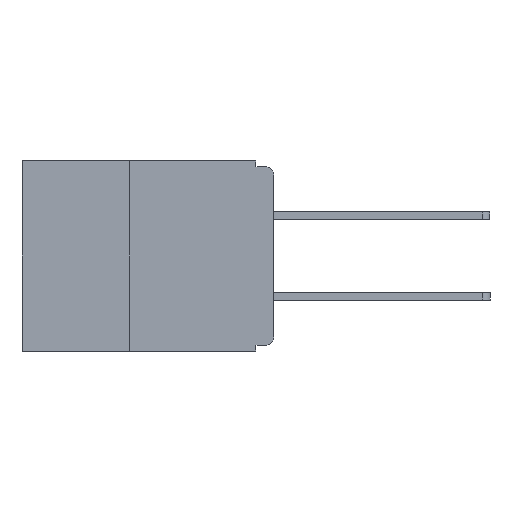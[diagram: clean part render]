
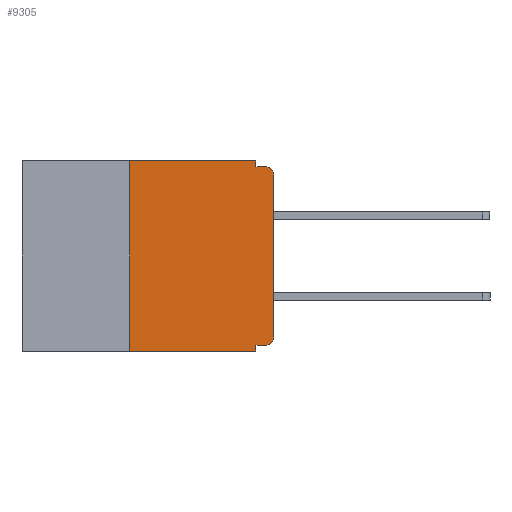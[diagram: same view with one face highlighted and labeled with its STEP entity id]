
A CAD part, left-side view. The second image highlights one B-rep face of the part: STEP entity #9305.
In plain terms, the highlighted planar face has unit normal (-1, 0, 0).
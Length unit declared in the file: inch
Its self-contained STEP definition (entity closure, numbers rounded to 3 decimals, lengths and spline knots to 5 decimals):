
#708 = CARTESIAN_POINT ( 'NONE',  ( 0., 0.437, -0.33 ) ) ;
#750 = CARTESIAN_POINT ( 'NONE',  ( 0., 0.25, 0. ) ) ;
#878 = DIRECTION ( 'NONE',  ( 0., -1., 0. ) ) ;
#1476 = CARTESIAN_POINT ( 'NONE',  ( 0., 0., -0.305 ) ) ;
#1498 = VERTEX_POINT ( 'NONE', #3776 ) ;
#1528 = LINE ( 'NONE', #10200, #16758 ) ;
#1760 = VERTEX_POINT ( 'NONE', #2878 ) ;
#1924 = EDGE_CURVE ( 'NONE', #11051, #5917, #13433, .T. ) ;
#2057 = VECTOR ( 'NONE', #4508, 39.37008 ) ;
#2262 = LINE ( 'NONE', #12941, #9927 ) ;
#2446 = CARTESIAN_POINT ( 'NONE',  ( 0., 0.015, -0.305 ) ) ;
#2624 = DIRECTION ( 'NONE',  ( 0., -1., 0. ) ) ;
#2639 = EDGE_CURVE ( 'NONE', #6317, #6076, #14489, .T. ) ;
#2843 = AXIS2_PLACEMENT_3D ( 'NONE', #13526, #4661, #14901 ) ;
#2878 = CARTESIAN_POINT ( 'NONE',  ( 0., 0.25, -0.33 ) ) ;
#2907 = CARTESIAN_POINT ( 'NONE',  ( 0., 0.031, 0. ) ) ;
#2910 = VERTEX_POINT ( 'NONE', #8600 ) ;
#3376 = LINE ( 'NONE', #13582, #10904 ) ;
#3776 = CARTESIAN_POINT ( 'NONE',  ( 0., 0., -0.025 ) ) ;
#4038 = DIRECTION ( 'NONE',  ( 0., 0., -1. ) ) ;
#4508 = DIRECTION ( 'NONE',  ( 0., 0., -1. ) ) ;
#4661 = DIRECTION ( 'NONE',  ( -1., 0., 0. ) ) ;
#4781 = ORIENTED_EDGE ( 'NONE', *, *, #14930, .T. ) ;
#5470 = VERTEX_POINT ( 'NONE', #12471 ) ;
#5583 = ORIENTED_EDGE ( 'NONE', *, *, #16730, .T. ) ;
#5917 = VERTEX_POINT ( 'NONE', #18524 ) ;
#6076 = VERTEX_POINT ( 'NONE', #16969 ) ;
#6317 = VERTEX_POINT ( 'NONE', #13900 ) ;
#6338 = EDGE_CURVE ( 'NONE', #6076, #2910, #3376, .T. ) ;
#6713 = CARTESIAN_POINT ( 'NONE',  ( 0., 0.25, -0.33 ) ) ;
#6873 = ORIENTED_EDGE ( 'NONE', *, *, #11763, .F. ) ;
#7220 = CARTESIAN_POINT ( 'NONE',  ( 0., 0.015, -0.01 ) ) ;
#7301 = EDGE_CURVE ( 'NONE', #1760, #2910, #16401, .T. ) ;
#7721 = ORIENTED_EDGE ( 'NONE', *, *, #2639, .F. ) ;
#8220 = DIRECTION ( 'NONE',  ( 0., 0., 1. ) ) ;
#8307 = ORIENTED_EDGE ( 'NONE', *, *, #6338, .F. ) ;
#8600 = CARTESIAN_POINT ( 'NONE',  ( 0., 0.031, -0.33 ) ) ;
#8856 = CIRCLE ( 'NONE', #2843, 0.015 ) ;
#8909 = CIRCLE ( 'NONE', #12575, 0.015 ) ;
#9287 = ORIENTED_EDGE ( 'NONE', *, *, #7301, .T. ) ;
#9305 = ADVANCED_FACE ( 'NONE', ( #16525 ), #10115, .F. ) ;
#9324 = VECTOR ( 'NONE', #878, 39.37008 ) ;
#9750 = DIRECTION ( 'NONE',  ( 0., 1., 0. ) ) ;
#9804 = DIRECTION ( 'NONE',  ( 0., 0., -1. ) ) ;
#9918 = VERTEX_POINT ( 'NONE', #7220 ) ;
#9927 = VECTOR ( 'NONE', #14334, 39.37008 ) ;
#9943 = DIRECTION ( 'NONE',  ( 1., 0., 0. ) ) ;
#10005 = CARTESIAN_POINT ( 'NONE',  ( 0., 0.437, 0. ) ) ;
#10115 = PLANE ( 'NONE',  #17469 ) ;
#10200 = CARTESIAN_POINT ( 'NONE',  ( 0., 0., -0.01 ) ) ;
#10269 = EDGE_CURVE ( 'NONE', #1760, #11051, #18314, .T. ) ;
#10552 = VECTOR ( 'NONE', #8220, 39.37008 ) ;
#10657 = ORIENTED_EDGE ( 'NONE', *, *, #1924, .F. ) ;
#10738 = CARTESIAN_POINT ( 'NONE',  ( 0., 0.437, 0. ) ) ;
#10904 = VECTOR ( 'NONE', #13400, 39.37008 ) ;
#11051 = VERTEX_POINT ( 'NONE', #750 ) ;
#11240 = EDGE_CURVE ( 'NONE', #5917, #5470, #14044, .T. ) ;
#11345 = VERTEX_POINT ( 'NONE', #1476 ) ;
#11763 = EDGE_CURVE ( 'NONE', #5470, #9918, #1528, .T. ) ;
#12134 = DIRECTION ( 'NONE',  ( 0., -1., 0. ) ) ;
#12471 = CARTESIAN_POINT ( 'NONE',  ( 0., 0.031, -0.01 ) ) ;
#12575 = AXIS2_PLACEMENT_3D ( 'NONE', #2446, #12997, #4038 ) ;
#12941 = CARTESIAN_POINT ( 'NONE',  ( 0., 0., 0. ) ) ;
#12997 = DIRECTION ( 'NONE',  ( -1., 0., 0. ) ) ;
#13006 = VECTOR ( 'NONE', #12134, 39.37008 ) ;
#13260 = ORIENTED_EDGE ( 'NONE', *, *, #10269, .F. ) ;
#13400 = DIRECTION ( 'NONE',  ( 0., 0., -1. ) ) ;
#13433 = LINE ( 'NONE', #10738, #13006 ) ;
#13526 = CARTESIAN_POINT ( 'NONE',  ( 0., 0.015, -0.025 ) ) ;
#13582 = CARTESIAN_POINT ( 'NONE',  ( 0., 0.031, -0.33 ) ) ;
#13629 = ORIENTED_EDGE ( 'NONE', *, *, #11240, .F. ) ;
#13755 = ORIENTED_EDGE ( 'NONE', *, *, #18131, .T. ) ;
#13900 = CARTESIAN_POINT ( 'NONE',  ( 0., 0.015, -0.32 ) ) ;
#14044 = LINE ( 'NONE', #2907, #2057 ) ;
#14334 = DIRECTION ( 'NONE',  ( 0., 0., 1. ) ) ;
#14489 = LINE ( 'NONE', #15088, #16794 ) ;
#14531 = EDGE_LOOP ( 'NONE', ( #13755, #5583, #6873, #13629, #10657, #13260, #9287, #8307, #7721, #4781 ) ) ;
#14901 = DIRECTION ( 'NONE',  ( 0., 0., -1. ) ) ;
#14930 = EDGE_CURVE ( 'NONE', #6317, #11345, #8909, .T. ) ;
#15088 = CARTESIAN_POINT ( 'NONE',  ( 0., 0., -0.32 ) ) ;
#16401 = LINE ( 'NONE', #708, #9324 ) ;
#16525 = FACE_OUTER_BOUND ( 'NONE', #14531, .T. ) ;
#16730 = EDGE_CURVE ( 'NONE', #1498, #9918, #8856, .T. ) ;
#16758 = VECTOR ( 'NONE', #2624, 39.37008 ) ;
#16794 = VECTOR ( 'NONE', #9750, 39.37008 ) ;
#16969 = CARTESIAN_POINT ( 'NONE',  ( 0., 0.031, -0.32 ) ) ;
#17469 = AXIS2_PLACEMENT_3D ( 'NONE', #10005, #9943, #9804 ) ;
#18131 = EDGE_CURVE ( 'NONE', #11345, #1498, #2262, .T. ) ;
#18314 = LINE ( 'NONE', #6713, #10552 ) ;
#18524 = CARTESIAN_POINT ( 'NONE',  ( 0., 0.031, 0. ) ) ;
